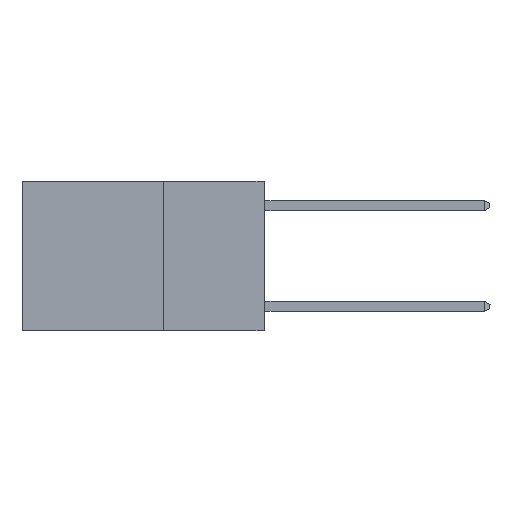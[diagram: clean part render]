
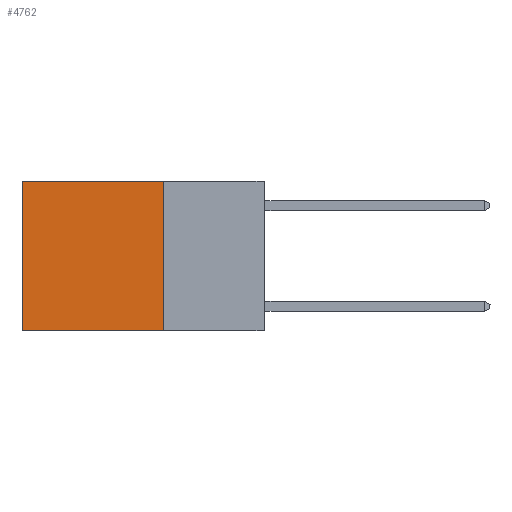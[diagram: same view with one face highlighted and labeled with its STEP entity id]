
A CAD part, left-side view. The second image highlights one B-rep face of the part: STEP entity #4762.
In plain terms, the highlighted planar face has unit normal (-1, 0, 0).
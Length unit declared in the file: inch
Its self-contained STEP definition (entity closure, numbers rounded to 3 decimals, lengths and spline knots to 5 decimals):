
#545 = LINE ( 'NONE', #8124, #11034 ) ;
#897 = DIRECTION ( 'NONE',  ( 0., 1., 0. ) ) ;
#1596 = EDGE_CURVE ( 'NONE', #13548, #10802, #12312, .T. ) ;
#2040 = DIRECTION ( 'NONE',  ( 1., 0., 0. ) ) ;
#2745 = LINE ( 'NONE', #11335, #6631 ) ;
#2804 = CARTESIAN_POINT ( 'NONE',  ( 0.2625, 0.6, 0. ) ) ;
#4049 = ORIENTED_EDGE ( 'NONE', *, *, #12882, .T. ) ;
#4762 = ADVANCED_FACE ( 'NONE', ( #10156 ), #9088, .F. ) ;
#5349 = DIRECTION ( 'NONE',  ( 0., 1., 0. ) ) ;
#5396 = EDGE_CURVE ( 'NONE', #10802, #11180, #12476, .T. ) ;
#5475 = CARTESIAN_POINT ( 'NONE',  ( 0.2625, 0.25, 0. ) ) ;
#6141 = CARTESIAN_POINT ( 'NONE',  ( 0.2625, 0.25, 0. ) ) ;
#6571 = ORIENTED_EDGE ( 'NONE', *, *, #1596, .F. ) ;
#6631 = VECTOR ( 'NONE', #897, 39.37008 ) ;
#7041 = AXIS2_PLACEMENT_3D ( 'NONE', #5475, #2040, #11301 ) ;
#7178 = VECTOR ( 'NONE', #5349, 39.37008 ) ;
#8124 = CARTESIAN_POINT ( 'NONE',  ( 0.2625, 0.6, 0. ) ) ;
#8332 = DIRECTION ( 'NONE',  ( 0., 0., -1. ) ) ;
#8925 = EDGE_LOOP ( 'NONE', ( #4049, #11294, #6571, #12643 ) ) ;
#9088 = PLANE ( 'NONE',  #7041 ) ;
#9333 = CARTESIAN_POINT ( 'NONE',  ( 0.2625, 0.25, -0.37 ) ) ;
#10110 = CARTESIAN_POINT ( 'NONE',  ( 0.2625, 0.25, -0.37 ) ) ;
#10156 = FACE_OUTER_BOUND ( 'NONE', #8925, .T. ) ;
#10802 = VERTEX_POINT ( 'NONE', #9333 ) ;
#11034 = VECTOR ( 'NONE', #12876, 39.37008 ) ;
#11180 = VERTEX_POINT ( 'NONE', #14542 ) ;
#11294 = ORIENTED_EDGE ( 'NONE', *, *, #5396, .F. ) ;
#11301 = DIRECTION ( 'NONE',  ( 0., 0., -1. ) ) ;
#11335 = CARTESIAN_POINT ( 'NONE',  ( 0.2625, 0.25, 0. ) ) ;
#11718 = CARTESIAN_POINT ( 'NONE',  ( 0.2625, 0.25, 0. ) ) ;
#12312 = LINE ( 'NONE', #11718, #13758 ) ;
#12476 = LINE ( 'NONE', #10110, #7178 ) ;
#12564 = VERTEX_POINT ( 'NONE', #2804 ) ;
#12643 = ORIENTED_EDGE ( 'NONE', *, *, #12763, .T. ) ;
#12763 = EDGE_CURVE ( 'NONE', #13548, #12564, #2745, .T. ) ;
#12876 = DIRECTION ( 'NONE',  ( 0., 0., -1. ) ) ;
#12882 = EDGE_CURVE ( 'NONE', #12564, #11180, #545, .T. ) ;
#13548 = VERTEX_POINT ( 'NONE', #6141 ) ;
#13758 = VECTOR ( 'NONE', #8332, 39.37008 ) ;
#14542 = CARTESIAN_POINT ( 'NONE',  ( 0.2625, 0.6, -0.37 ) ) ;
